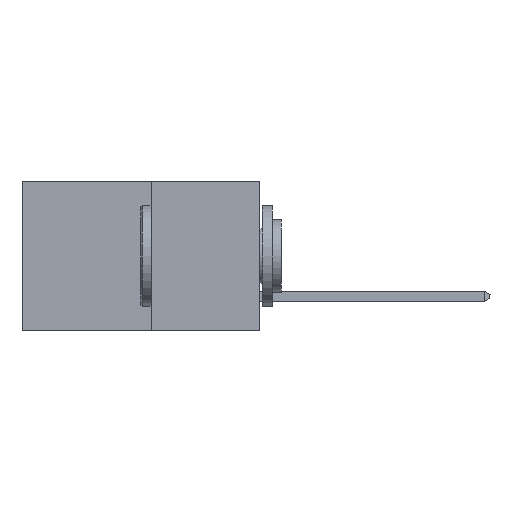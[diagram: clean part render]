
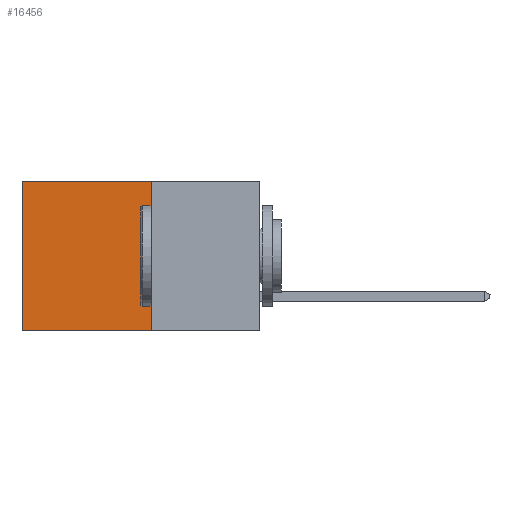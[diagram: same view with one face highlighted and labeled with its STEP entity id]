
A CAD part, left-side view. The second image highlights one B-rep face of the part: STEP entity #16456.
In plain terms, the highlighted planar face has unit normal (-1, 0, 0).
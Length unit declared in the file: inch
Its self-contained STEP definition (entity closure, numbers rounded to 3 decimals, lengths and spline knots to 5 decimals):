
#29 = VERTEX_POINT ( 'NONE', #21858 ) ;
#169 = LINE ( 'NONE', #16360, #17146 ) ;
#1394 = AXIS2_PLACEMENT_3D ( 'NONE', #17028, #5918, #21462 ) ;
#1990 = EDGE_CURVE ( 'NONE', #20536, #10278, #15866, .T. ) ;
#2894 = EDGE_CURVE ( 'NONE', #10278, #29, #15520, .T. ) ;
#3420 = CARTESIAN_POINT ( 'NONE',  ( 0.277, 0.27, 0. ) ) ;
#3718 = PLANE ( 'NONE',  #1394 ) ;
#3733 = CARTESIAN_POINT ( 'NONE',  ( 0.277, 0.59, -0.37 ) ) ;
#3883 = EDGE_CURVE ( 'NONE', #20536, #23007, #169, .T. ) ;
#4553 = LINE ( 'NONE', #13049, #15719 ) ;
#4565 = CARTESIAN_POINT ( 'NONE',  ( 0.277, 0.27, -0.37 ) ) ;
#5174 = EDGE_CURVE ( 'NONE', #23007, #29, #4553, .T. ) ;
#5918 = DIRECTION ( 'NONE',  ( 1., 0., 0. ) ) ;
#8025 = DIRECTION ( 'NONE',  ( 0., 1., 0. ) ) ;
#9899 = VECTOR ( 'NONE', #14541, 39.37008 ) ;
#10278 = VERTEX_POINT ( 'NONE', #11131 ) ;
#11131 = CARTESIAN_POINT ( 'NONE',  ( 0.277, 0.59, 0. ) ) ;
#12619 = DIRECTION ( 'NONE',  ( 0., 0., -1. ) ) ;
#13049 = CARTESIAN_POINT ( 'NONE',  ( 0.277, 0.27, -0.37 ) ) ;
#14541 = DIRECTION ( 'NONE',  ( 0., 1., 0. ) ) ;
#14811 = VECTOR ( 'NONE', #17893, 39.37008 ) ;
#15520 = LINE ( 'NONE', #3733, #14811 ) ;
#15719 = VECTOR ( 'NONE', #8025, 39.37008 ) ;
#15866 = LINE ( 'NONE', #3420, #9899 ) ;
#16360 = CARTESIAN_POINT ( 'NONE',  ( 0.277, 0.27, -0.37 ) ) ;
#16456 = ADVANCED_FACE ( 'NONE', ( #21363 ), #3718, .F. ) ;
#17028 = CARTESIAN_POINT ( 'NONE',  ( 0.277, 0.27, -0.37 ) ) ;
#17146 = VECTOR ( 'NONE', #12619, 39.37008 ) ;
#17377 = ORIENTED_EDGE ( 'NONE', *, *, #5174, .F. ) ;
#17893 = DIRECTION ( 'NONE',  ( 0., 0., -1. ) ) ;
#19810 = ORIENTED_EDGE ( 'NONE', *, *, #2894, .T. ) ;
#20536 = VERTEX_POINT ( 'NONE', #24764 ) ;
#21363 = FACE_OUTER_BOUND ( 'NONE', #24051, .T. ) ;
#21462 = DIRECTION ( 'NONE',  ( 0., 0., -1. ) ) ;
#21858 = CARTESIAN_POINT ( 'NONE',  ( 0.277, 0.59, -0.37 ) ) ;
#23007 = VERTEX_POINT ( 'NONE', #4565 ) ;
#24051 = EDGE_LOOP ( 'NONE', ( #19810, #17377, #25869, #25237 ) ) ;
#24764 = CARTESIAN_POINT ( 'NONE',  ( 0.277, 0.27, 0. ) ) ;
#25237 = ORIENTED_EDGE ( 'NONE', *, *, #1990, .T. ) ;
#25869 = ORIENTED_EDGE ( 'NONE', *, *, #3883, .F. ) ;
